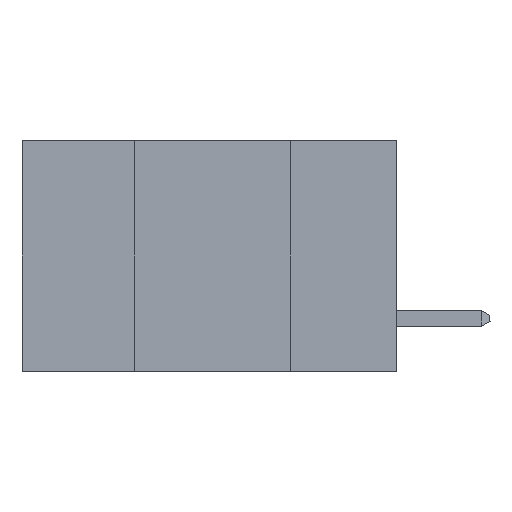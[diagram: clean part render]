
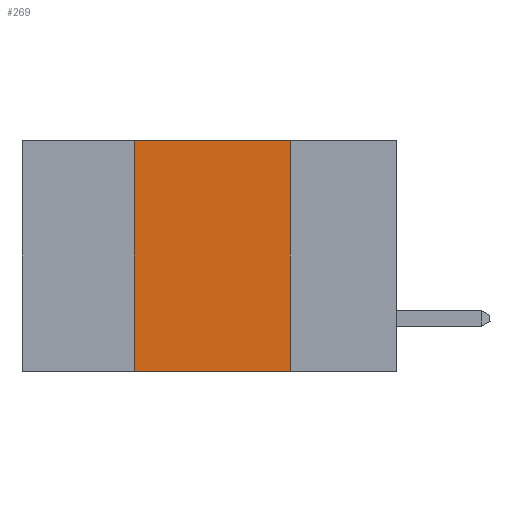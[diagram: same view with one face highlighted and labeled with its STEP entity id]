
A CAD part, left-side view. The second image highlights one B-rep face of the part: STEP entity #269.
In plain terms, the highlighted planar face has unit normal (-1, 0, 0).
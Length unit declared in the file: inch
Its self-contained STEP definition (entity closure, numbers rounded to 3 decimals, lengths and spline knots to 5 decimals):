
#269 = ADVANCED_FACE ( 'NONE', ( #20393 ), #20569, .F. ) ;
#304 = VERTEX_POINT ( 'NONE', #22148 ) ;
#362 = LINE ( 'NONE', #17591, #10929 ) ;
#628 = CARTESIAN_POINT ( 'NONE',  ( 0., 0.42, 0. ) ) ;
#1301 = VECTOR ( 'NONE', #5952, 39.37008 ) ;
#2030 = VERTEX_POINT ( 'NONE', #19956 ) ;
#3505 = EDGE_LOOP ( 'NONE', ( #19096, #24796, #7678, #6673 ) ) ;
#4825 = EDGE_CURVE ( 'NONE', #304, #11664, #12708, .T. ) ;
#5495 = AXIS2_PLACEMENT_3D ( 'NONE', #20054, #12890, #15339 ) ;
#5952 = DIRECTION ( 'NONE',  ( 0., -1., 0. ) ) ;
#6673 = ORIENTED_EDGE ( 'NONE', *, *, #6758, .T. ) ;
#6758 = EDGE_CURVE ( 'NONE', #2030, #11664, #362, .T. ) ;
#7611 = LINE ( 'NONE', #22674, #1301 ) ;
#7678 = ORIENTED_EDGE ( 'NONE', *, *, #16197, .F. ) ;
#7915 = LINE ( 'NONE', #628, #18372 ) ;
#8532 = CARTESIAN_POINT ( 'NONE',  ( 0., 0.17, -0.37 ) ) ;
#8897 = EDGE_CURVE ( 'NONE', #26160, #304, #7611, .T. ) ;
#10929 = VECTOR ( 'NONE', #25921, 39.37008 ) ;
#10958 = CARTESIAN_POINT ( 'NONE',  ( 0., 0.42, 0. ) ) ;
#11664 = VERTEX_POINT ( 'NONE', #8532 ) ;
#12708 = LINE ( 'NONE', #15363, #23157 ) ;
#12890 = DIRECTION ( 'NONE',  ( 1., 0., 0. ) ) ;
#15339 = DIRECTION ( 'NONE',  ( 0., 0., -1. ) ) ;
#15363 = CARTESIAN_POINT ( 'NONE',  ( 0., 0.17, 0. ) ) ;
#16197 = EDGE_CURVE ( 'NONE', #2030, #26160, #7915, .T. ) ;
#17466 = DIRECTION ( 'NONE',  ( 0., 0., 1. ) ) ;
#17591 = CARTESIAN_POINT ( 'NONE',  ( 0., 0.6, -0.37 ) ) ;
#18372 = VECTOR ( 'NONE', #17466, 39.37008 ) ;
#19096 = ORIENTED_EDGE ( 'NONE', *, *, #4825, .F. ) ;
#19956 = CARTESIAN_POINT ( 'NONE',  ( 0., 0.42, -0.37 ) ) ;
#20054 = CARTESIAN_POINT ( 'NONE',  ( 0., 0.6, 0. ) ) ;
#20393 = FACE_OUTER_BOUND ( 'NONE', #3505, .T. ) ;
#20569 = PLANE ( 'NONE',  #5495 ) ;
#22147 = DIRECTION ( 'NONE',  ( 0., 0., -1. ) ) ;
#22148 = CARTESIAN_POINT ( 'NONE',  ( 0., 0.17, 0. ) ) ;
#22674 = CARTESIAN_POINT ( 'NONE',  ( 0., 0.6, 0. ) ) ;
#23157 = VECTOR ( 'NONE', #22147, 39.37008 ) ;
#24796 = ORIENTED_EDGE ( 'NONE', *, *, #8897, .F. ) ;
#25921 = DIRECTION ( 'NONE',  ( 0., -1., 0. ) ) ;
#26160 = VERTEX_POINT ( 'NONE', #10958 ) ;
